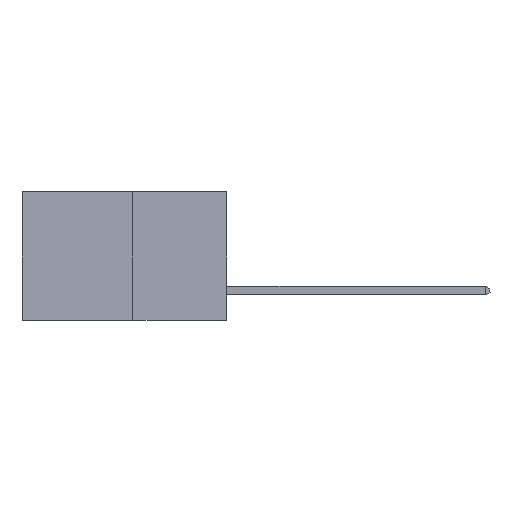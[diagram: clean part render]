
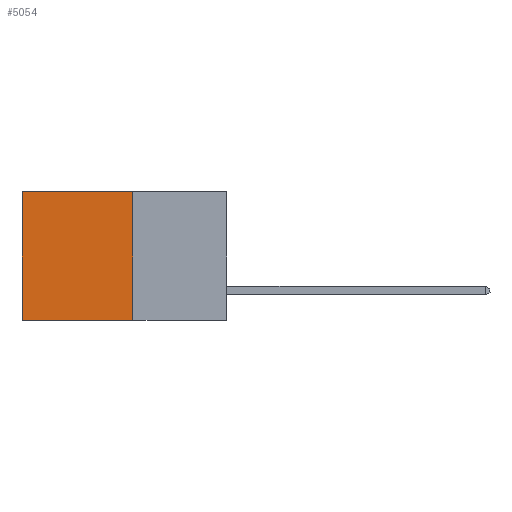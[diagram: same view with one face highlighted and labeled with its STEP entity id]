
A CAD part, left-side view. The second image highlights one B-rep face of the part: STEP entity #5054.
In plain terms, the highlighted planar face has unit normal (-1, 0, 0).
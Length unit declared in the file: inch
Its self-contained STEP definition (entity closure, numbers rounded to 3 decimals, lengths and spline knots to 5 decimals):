
#288 = EDGE_CURVE ( 'NONE', #954, #4977, #931, .T. ) ;
#653 = DIRECTION ( 'NONE',  ( 0., 0., -1. ) ) ;
#931 = LINE ( 'NONE', #13360, #9465 ) ;
#954 = VERTEX_POINT ( 'NONE', #6655 ) ;
#1896 = CARTESIAN_POINT ( 'NONE',  ( 0.277, 0.59, -0.37 ) ) ;
#1985 = EDGE_CURVE ( 'NONE', #4977, #9282, #2590, .T. ) ;
#2108 = PLANE ( 'NONE',  #14214 ) ;
#2156 = CARTESIAN_POINT ( 'NONE',  ( 0.277, 0.27, -0.37 ) ) ;
#2421 = EDGE_CURVE ( 'NONE', #13638, #9282, #9346, .T. ) ;
#2590 = LINE ( 'NONE', #12947, #5496 ) ;
#3204 = DIRECTION ( 'NONE',  ( 0., 1., 0. ) ) ;
#3767 = ORIENTED_EDGE ( 'NONE', *, *, #2421, .F. ) ;
#4955 = VECTOR ( 'NONE', #653, 39.37008 ) ;
#4977 = VERTEX_POINT ( 'NONE', #12658 ) ;
#5007 = ORIENTED_EDGE ( 'NONE', *, *, #288, .T. ) ;
#5054 = ADVANCED_FACE ( 'NONE', ( #13677 ), #2108, .F. ) ;
#5496 = VECTOR ( 'NONE', #12472, 39.37008 ) ;
#6655 = CARTESIAN_POINT ( 'NONE',  ( 0.277, 0.27, 0. ) ) ;
#7955 = ORIENTED_EDGE ( 'NONE', *, *, #1985, .T. ) ;
#9282 = VERTEX_POINT ( 'NONE', #1896 ) ;
#9346 = LINE ( 'NONE', #12526, #14922 ) ;
#9465 = VECTOR ( 'NONE', #10734, 39.37008 ) ;
#10135 = DIRECTION ( 'NONE',  ( 0., 0., -1. ) ) ;
#10734 = DIRECTION ( 'NONE',  ( 0., 1., 0. ) ) ;
#12471 = ORIENTED_EDGE ( 'NONE', *, *, #13391, .F. ) ;
#12472 = DIRECTION ( 'NONE',  ( 0., 0., -1. ) ) ;
#12526 = CARTESIAN_POINT ( 'NONE',  ( 0.277, 0.27, -0.37 ) ) ;
#12658 = CARTESIAN_POINT ( 'NONE',  ( 0.277, 0.59, 0. ) ) ;
#12947 = CARTESIAN_POINT ( 'NONE',  ( 0.277, 0.59, -0.37 ) ) ;
#12969 = DIRECTION ( 'NONE',  ( 1., 0., 0. ) ) ;
#13360 = CARTESIAN_POINT ( 'NONE',  ( 0.277, 0.27, 0. ) ) ;
#13391 = EDGE_CURVE ( 'NONE', #954, #13638, #14117, .T. ) ;
#13638 = VERTEX_POINT ( 'NONE', #14124 ) ;
#13677 = FACE_OUTER_BOUND ( 'NONE', #14204, .T. ) ;
#14117 = LINE ( 'NONE', #14731, #4955 ) ;
#14124 = CARTESIAN_POINT ( 'NONE',  ( 0.277, 0.27, -0.37 ) ) ;
#14204 = EDGE_LOOP ( 'NONE', ( #7955, #3767, #12471, #5007 ) ) ;
#14214 = AXIS2_PLACEMENT_3D ( 'NONE', #2156, #12969, #10135 ) ;
#14731 = CARTESIAN_POINT ( 'NONE',  ( 0.277, 0.27, -0.37 ) ) ;
#14922 = VECTOR ( 'NONE', #3204, 39.37008 ) ;
